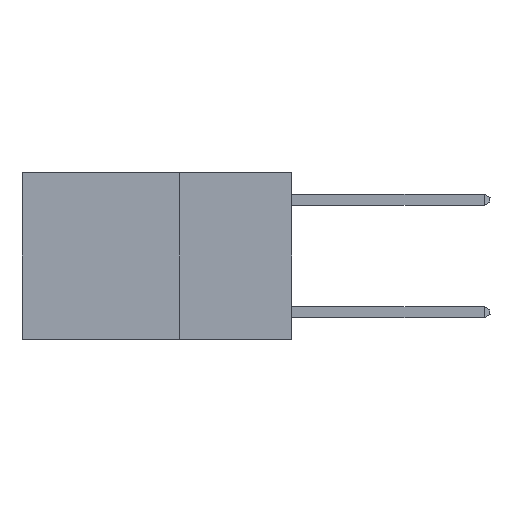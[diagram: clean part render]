
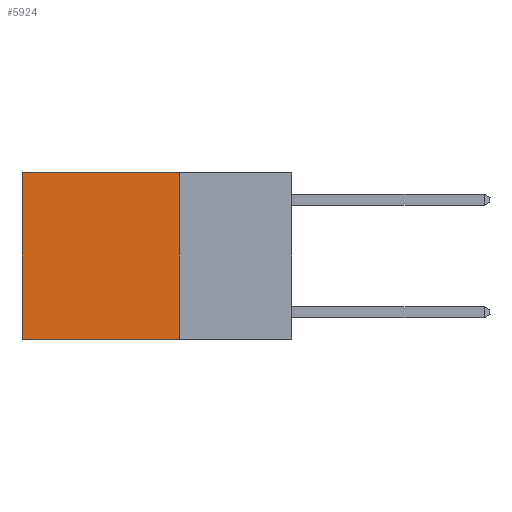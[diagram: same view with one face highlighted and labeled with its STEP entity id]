
A CAD part, left-side view. The second image highlights one B-rep face of the part: STEP entity #5924.
In plain terms, the highlighted planar face has unit normal (-1, 0, 0).
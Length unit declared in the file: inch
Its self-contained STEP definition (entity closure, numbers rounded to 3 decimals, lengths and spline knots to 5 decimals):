
#544 = EDGE_CURVE ( 'NONE', #6335, #5537, #15336, .T. ) ;
#703 = DIRECTION ( 'NONE',  ( 0., 0., -1. ) ) ;
#792 = VECTOR ( 'NONE', #7984, 39.37008 ) ;
#964 = VECTOR ( 'NONE', #14583, 39.37008 ) ;
#1319 = FACE_OUTER_BOUND ( 'NONE', #11449, .T. ) ;
#3014 = CARTESIAN_POINT ( 'NONE',  ( 0.2625, 0.25, 0. ) ) ;
#5367 = VECTOR ( 'NONE', #12713, 39.37008 ) ;
#5537 = VERTEX_POINT ( 'NONE', #8930 ) ;
#5603 = CARTESIAN_POINT ( 'NONE',  ( 0.2625, 0.25, -0.37 ) ) ;
#5924 = ADVANCED_FACE ( 'NONE', ( #1319 ), #12958, .F. ) ;
#6335 = VERTEX_POINT ( 'NONE', #7877 ) ;
#7152 = DIRECTION ( 'NONE',  ( 0., 0., -1. ) ) ;
#7374 = CARTESIAN_POINT ( 'NONE',  ( 0.2625, 0.25, 0. ) ) ;
#7778 = CARTESIAN_POINT ( 'NONE',  ( 0.2625, 0.6, 0. ) ) ;
#7877 = CARTESIAN_POINT ( 'NONE',  ( 0.2625, 0.6, 0. ) ) ;
#7984 = DIRECTION ( 'NONE',  ( 0., 1., 0. ) ) ;
#8158 = VERTEX_POINT ( 'NONE', #12336 ) ;
#8317 = EDGE_CURVE ( 'NONE', #15996, #8158, #15712, .T. ) ;
#8458 = DIRECTION ( 'NONE',  ( 1., 0., 0. ) ) ;
#8811 = ORIENTED_EDGE ( 'NONE', *, *, #8317, .F. ) ;
#8930 = CARTESIAN_POINT ( 'NONE',  ( 0.2625, 0.6, -0.37 ) ) ;
#9695 = EDGE_CURVE ( 'NONE', #8158, #5537, #11314, .T. ) ;
#10068 = ORIENTED_EDGE ( 'NONE', *, *, #17959, .T. ) ;
#10514 = LINE ( 'NONE', #16424, #792 ) ;
#10552 = ORIENTED_EDGE ( 'NONE', *, *, #9695, .F. ) ;
#11314 = LINE ( 'NONE', #5603, #964 ) ;
#11449 = EDGE_LOOP ( 'NONE', ( #15334, #10552, #8811, #10068 ) ) ;
#12336 = CARTESIAN_POINT ( 'NONE',  ( 0.2625, 0.25, -0.37 ) ) ;
#12713 = DIRECTION ( 'NONE',  ( 0., 0., -1. ) ) ;
#12958 = PLANE ( 'NONE',  #15805 ) ;
#13075 = CARTESIAN_POINT ( 'NONE',  ( 0.2625, 0.25, 0. ) ) ;
#14583 = DIRECTION ( 'NONE',  ( 0., 1., 0. ) ) ;
#15334 = ORIENTED_EDGE ( 'NONE', *, *, #544, .T. ) ;
#15336 = LINE ( 'NONE', #7778, #16794 ) ;
#15712 = LINE ( 'NONE', #7374, #5367 ) ;
#15805 = AXIS2_PLACEMENT_3D ( 'NONE', #3014, #8458, #7152 ) ;
#15996 = VERTEX_POINT ( 'NONE', #13075 ) ;
#16424 = CARTESIAN_POINT ( 'NONE',  ( 0.2625, 0.25, 0. ) ) ;
#16794 = VECTOR ( 'NONE', #703, 39.37008 ) ;
#17959 = EDGE_CURVE ( 'NONE', #15996, #6335, #10514, .T. ) ;
